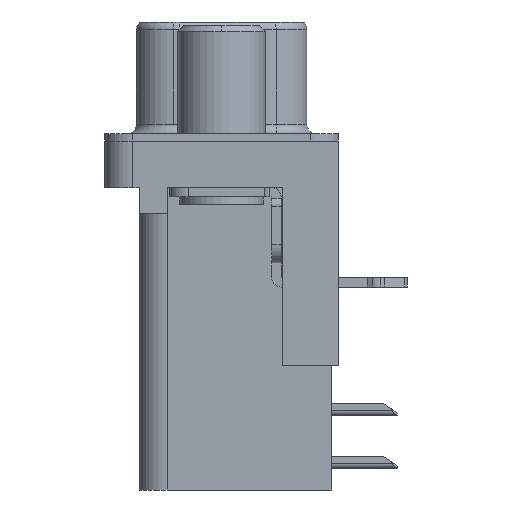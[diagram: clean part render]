
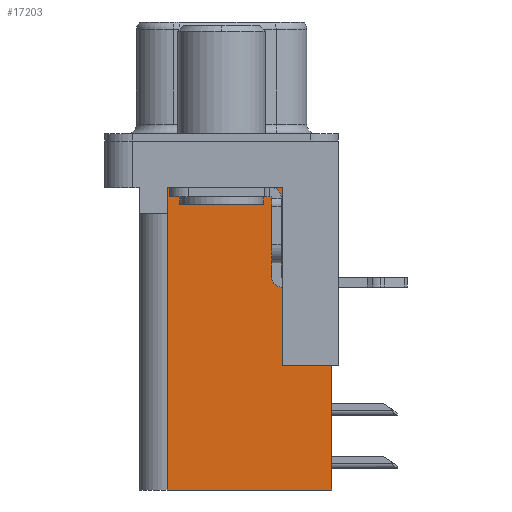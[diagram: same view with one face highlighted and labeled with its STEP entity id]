
A CAD part, left-side view. The second image highlights one B-rep face of the part: STEP entity #17203.
In plain terms, the highlighted planar face has unit normal (-1, 0, 0).
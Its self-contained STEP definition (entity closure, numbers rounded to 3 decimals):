
#638 = LINE ( 'NONE', #15843, #700 ) ;
#685 = CARTESIAN_POINT ( 'NONE',  ( 3.765, -5.925, -18.76 ) ) ;
#700 = VECTOR ( 'NONE', #5215, 1000. ) ;
#975 = DIRECTION ( 'NONE',  ( 0., 1., 0. ) ) ;
#1429 = CARTESIAN_POINT ( 'NONE',  ( 3.765, -3.295, -18.76 ) ) ;
#1564 = ORIENTED_EDGE ( 'NONE', *, *, #16632, .F. ) ;
#1899 = VECTOR ( 'NONE', #11975, 1000. ) ;
#1916 = LINE ( 'NONE', #5795, #1899 ) ;
#2011 = VECTOR ( 'NONE', #14953, 1000. ) ;
#2286 = FACE_OUTER_BOUND ( 'NONE', #3888, .T. ) ;
#2541 = CARTESIAN_POINT ( 'NONE',  ( 3.765, 2.925, -18.76 ) ) ;
#3275 = CARTESIAN_POINT ( 'NONE',  ( 3.765, -5.925, -12.05 ) ) ;
#3888 = EDGE_LOOP ( 'NONE', ( #10672, #7046, #5199, #1564, #12479, #18899, #14547, #5337 ) ) ;
#4246 = CARTESIAN_POINT ( 'NONE',  ( 3.765, 2.895, -2.5 ) ) ;
#4358 = VECTOR ( 'NONE', #4613, 1000. ) ;
#4377 = LINE ( 'NONE', #9300, #4358 ) ;
#4613 = DIRECTION ( 'NONE',  ( 0., 0., 1. ) ) ;
#5199 = ORIENTED_EDGE ( 'NONE', *, *, #5475, .T. ) ;
#5215 = DIRECTION ( 'NONE',  ( 0., 0., -1. ) ) ;
#5337 = ORIENTED_EDGE ( 'NONE', *, *, #17976, .T. ) ;
#5338 = VECTOR ( 'NONE', #16762, 1000. ) ;
#5475 = EDGE_CURVE ( 'NONE', #10520, #15876, #5483, .T. ) ;
#5483 = LINE ( 'NONE', #16657, #5338 ) ;
#5795 = CARTESIAN_POINT ( 'NONE',  ( 3.765, -3.295, -18.76 ) ) ;
#5866 = CARTESIAN_POINT ( 'NONE',  ( 3.765, 2.895, -3.9 ) ) ;
#7046 = ORIENTED_EDGE ( 'NONE', *, *, #18749, .T. ) ;
#7308 = CARTESIAN_POINT ( 'NONE',  ( 3.765, -3.295, -18.76 ) ) ;
#7895 = VERTEX_POINT ( 'NONE', #4246 ) ;
#8971 = CARTESIAN_POINT ( 'NONE',  ( 3.765, -6.295, -12.05 ) ) ;
#9006 = DIRECTION ( 'NONE',  ( 0., 0., -1. ) ) ;
#9129 = AXIS2_PLACEMENT_3D ( 'NONE', #7308, #10402, #975 ) ;
#9300 = CARTESIAN_POINT ( 'NONE',  ( 3.765, 2.925, -18.76 ) ) ;
#9379 = EDGE_CURVE ( 'NONE', #9722, #7895, #10404, .T. ) ;
#9722 = VERTEX_POINT ( 'NONE', #11617 ) ;
#10288 = VECTOR ( 'NONE', #17886, 1000. ) ;
#10402 = DIRECTION ( 'NONE',  ( 1., 0., 0. ) ) ;
#10404 = LINE ( 'NONE', #10497, #10288 ) ;
#10497 = CARTESIAN_POINT ( 'NONE',  ( 3.765, -3.295, -2.5 ) ) ;
#10520 = VERTEX_POINT ( 'NONE', #11901 ) ;
#10672 = ORIENTED_EDGE ( 'NONE', *, *, #9379, .T. ) ;
#11617 = CARTESIAN_POINT ( 'NONE',  ( 3.765, -3.295, -2.5 ) ) ;
#11901 = CARTESIAN_POINT ( 'NONE',  ( 3.765, 2.895, -3.9 ) ) ;
#11926 = CARTESIAN_POINT ( 'NONE',  ( 3.765, -3.295, -12.05 ) ) ;
#11975 = DIRECTION ( 'NONE',  ( 0., 1., 0. ) ) ;
#12479 = ORIENTED_EDGE ( 'NONE', *, *, #17263, .F. ) ;
#12557 = VERTEX_POINT ( 'NONE', #2541 ) ;
#13127 = VERTEX_POINT ( 'NONE', #3275 ) ;
#14547 = ORIENTED_EDGE ( 'NONE', *, *, #17831, .T. ) ;
#14881 = CARTESIAN_POINT ( 'NONE',  ( 3.765, 2.925, -3.9 ) ) ;
#14913 = LINE ( 'NONE', #5866, #14948 ) ;
#14948 = VECTOR ( 'NONE', #9006, 1000. ) ;
#14953 = DIRECTION ( 'NONE',  ( 0., 1., 0. ) ) ;
#15321 = DIRECTION ( 'NONE',  ( 0., 0., 1. ) ) ;
#15777 = VERTEX_POINT ( 'NONE', #685 ) ;
#15843 = CARTESIAN_POINT ( 'NONE',  ( 3.765, -5.925, -2. ) ) ;
#15876 = VERTEX_POINT ( 'NONE', #14881 ) ;
#16407 = VERTEX_POINT ( 'NONE', #11926 ) ;
#16632 = EDGE_CURVE ( 'NONE', #12557, #15876, #4377, .T. ) ;
#16657 = CARTESIAN_POINT ( 'NONE',  ( 3.765, 0., -3.9 ) ) ;
#16762 = DIRECTION ( 'NONE',  ( 0., 1., 0. ) ) ;
#17203 = ADVANCED_FACE ( 'NONE', ( #2286 ), #19362, .F. ) ;
#17263 = EDGE_CURVE ( 'NONE', #15777, #12557, #1916, .T. ) ;
#17629 = EDGE_CURVE ( 'NONE', #13127, #15777, #638, .T. ) ;
#17831 = EDGE_CURVE ( 'NONE', #13127, #16407, #18365, .T. ) ;
#17886 = DIRECTION ( 'NONE',  ( 0., 1., 0. ) ) ;
#17976 = EDGE_CURVE ( 'NONE', #16407, #9722, #18566, .T. ) ;
#18365 = LINE ( 'NONE', #8971, #2011 ) ;
#18442 = VECTOR ( 'NONE', #15321, 1000. ) ;
#18566 = LINE ( 'NONE', #1429, #18442 ) ;
#18749 = EDGE_CURVE ( 'NONE', #7895, #10520, #14913, .T. ) ;
#18899 = ORIENTED_EDGE ( 'NONE', *, *, #17629, .F. ) ;
#19362 = PLANE ( 'NONE',  #9129 ) ;
